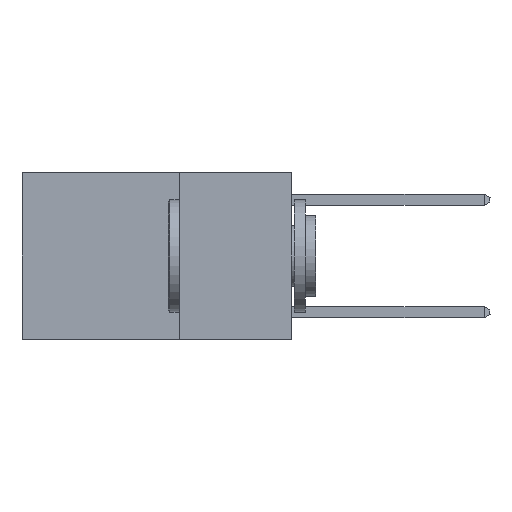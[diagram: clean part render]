
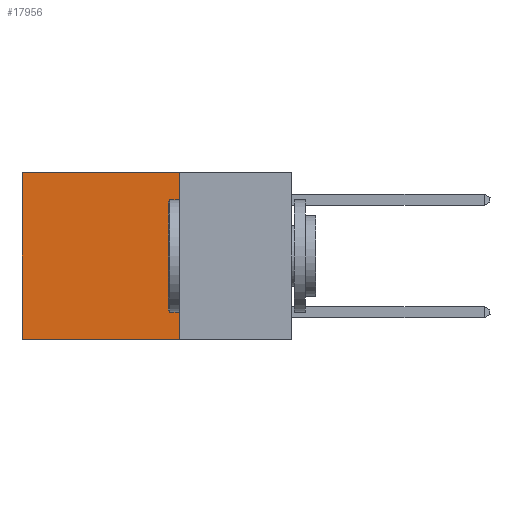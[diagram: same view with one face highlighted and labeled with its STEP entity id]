
A CAD part, left-side view. The second image highlights one B-rep face of the part: STEP entity #17956.
In plain terms, the highlighted planar face has unit normal (-1, 0, 0).
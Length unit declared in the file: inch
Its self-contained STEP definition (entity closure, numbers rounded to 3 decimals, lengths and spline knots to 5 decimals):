
#1707 = EDGE_CURVE ( 'NONE', #14997, #6875, #20851, .T. ) ;
#1790 = ORIENTED_EDGE ( 'NONE', *, *, #1707, .F. ) ;
#2355 = DIRECTION ( 'NONE',  ( 0., 1., 0. ) ) ;
#3179 = EDGE_CURVE ( 'NONE', #13617, #6875, #14064, .T. ) ;
#3664 = DIRECTION ( 'NONE',  ( 0., 1., 0. ) ) ;
#3972 = VECTOR ( 'NONE', #2355, 39.37008 ) ;
#4948 = FACE_OUTER_BOUND ( 'NONE', #16587, .T. ) ;
#5127 = CARTESIAN_POINT ( 'NONE',  ( 0.2625, 0.25, 0. ) ) ;
#6377 = CARTESIAN_POINT ( 'NONE',  ( 0.2625, 0.25, 0. ) ) ;
#6503 = PLANE ( 'NONE',  #19908 ) ;
#6774 = VECTOR ( 'NONE', #8790, 39.37008 ) ;
#6875 = VERTEX_POINT ( 'NONE', #9858 ) ;
#7027 = DIRECTION ( 'NONE',  ( 0., 0., -1. ) ) ;
#8790 = DIRECTION ( 'NONE',  ( 0., 0., -1. ) ) ;
#9858 = CARTESIAN_POINT ( 'NONE',  ( 0.2625, 0.6, -0.37 ) ) ;
#10344 = LINE ( 'NONE', #15415, #21591 ) ;
#10594 = LINE ( 'NONE', #17480, #3972 ) ;
#12052 = CARTESIAN_POINT ( 'NONE',  ( 0.2625, 0.25, -0.37 ) ) ;
#12777 = CARTESIAN_POINT ( 'NONE',  ( 0.2625, 0.25, -0.37 ) ) ;
#13617 = VERTEX_POINT ( 'NONE', #19470 ) ;
#14064 = LINE ( 'NONE', #15847, #6774 ) ;
#14746 = DIRECTION ( 'NONE',  ( 1., 0., 0. ) ) ;
#14997 = VERTEX_POINT ( 'NONE', #12777 ) ;
#15415 = CARTESIAN_POINT ( 'NONE',  ( 0.2625, 0.25, 0. ) ) ;
#15754 = VERTEX_POINT ( 'NONE', #5127 ) ;
#15847 = CARTESIAN_POINT ( 'NONE',  ( 0.2625, 0.6, 0. ) ) ;
#15878 = EDGE_CURVE ( 'NONE', #15754, #13617, #10594, .T. ) ;
#16587 = EDGE_LOOP ( 'NONE', ( #21669, #1790, #19803, #20788 ) ) ;
#17480 = CARTESIAN_POINT ( 'NONE',  ( 0.2625, 0.25, 0. ) ) ;
#17956 = ADVANCED_FACE ( 'NONE', ( #4948 ), #6503, .F. ) ;
#19426 = EDGE_CURVE ( 'NONE', #15754, #14997, #10344, .T. ) ;
#19470 = CARTESIAN_POINT ( 'NONE',  ( 0.2625, 0.6, 0. ) ) ;
#19803 = ORIENTED_EDGE ( 'NONE', *, *, #19426, .F. ) ;
#19908 = AXIS2_PLACEMENT_3D ( 'NONE', #6377, #14746, #21477 ) ;
#20254 = VECTOR ( 'NONE', #3664, 39.37008 ) ;
#20788 = ORIENTED_EDGE ( 'NONE', *, *, #15878, .T. ) ;
#20851 = LINE ( 'NONE', #12052, #20254 ) ;
#21477 = DIRECTION ( 'NONE',  ( 0., 0., -1. ) ) ;
#21591 = VECTOR ( 'NONE', #7027, 39.37008 ) ;
#21669 = ORIENTED_EDGE ( 'NONE', *, *, #3179, .T. ) ;
